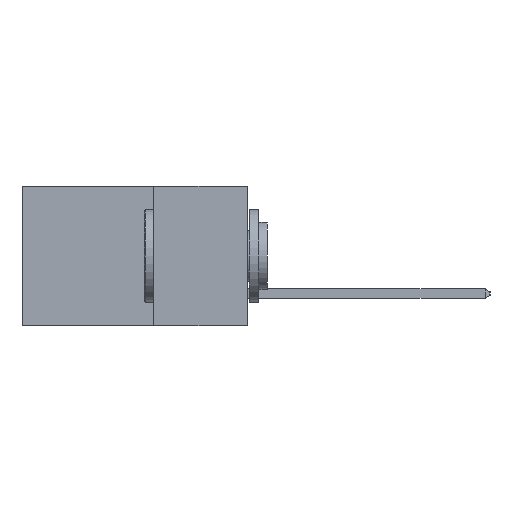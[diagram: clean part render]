
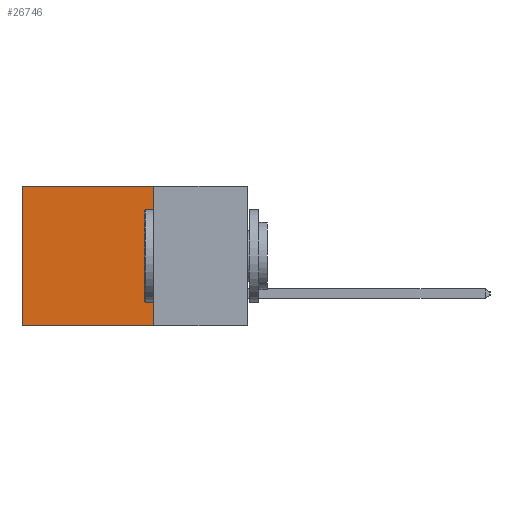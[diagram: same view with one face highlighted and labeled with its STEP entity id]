
A CAD part, left-side view. The second image highlights one B-rep face of the part: STEP entity #26746.
In plain terms, the highlighted planar face has unit normal (-1, 0, 0).
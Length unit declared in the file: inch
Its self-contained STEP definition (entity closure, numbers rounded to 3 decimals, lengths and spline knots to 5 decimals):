
#23 = VECTOR ( 'NONE', #11287, 39.37008 ) ;
#292 = EDGE_CURVE ( 'NONE', #16290, #5317, #12452, .T. ) ;
#1235 = FACE_OUTER_BOUND ( 'NONE', #13264, .T. ) ;
#2104 = CARTESIAN_POINT ( 'NONE',  ( 0.298, 0.6, 0. ) ) ;
#3529 = AXIS2_PLACEMENT_3D ( 'NONE', #7852, #22673, #10129 ) ;
#3675 = ORIENTED_EDGE ( 'NONE', *, *, #27439, .T. ) ;
#3745 = CARTESIAN_POINT ( 'NONE',  ( 0.298, 0.25, 0. ) ) ;
#4123 = VERTEX_POINT ( 'NONE', #21171 ) ;
#5091 = CARTESIAN_POINT ( 'NONE',  ( 0.298, 0.25, 0. ) ) ;
#5317 = VERTEX_POINT ( 'NONE', #16484 ) ;
#7852 = CARTESIAN_POINT ( 'NONE',  ( 0.298, 0.25, 0. ) ) ;
#8491 = CARTESIAN_POINT ( 'NONE',  ( 0.298, 0.25, -0.37 ) ) ;
#8669 = CARTESIAN_POINT ( 'NONE',  ( 0.298, 0.6, 0. ) ) ;
#10129 = DIRECTION ( 'NONE',  ( 0., 0., -1. ) ) ;
#10867 = DIRECTION ( 'NONE',  ( 0., 0., -1. ) ) ;
#11287 = DIRECTION ( 'NONE',  ( 0., 1., 0. ) ) ;
#12452 = LINE ( 'NONE', #8491, #23 ) ;
#12669 = LINE ( 'NONE', #8669, #23038 ) ;
#13264 = EDGE_LOOP ( 'NONE', ( #13481, #19899, #25701, #3675 ) ) ;
#13481 = ORIENTED_EDGE ( 'NONE', *, *, #18320, .T. ) ;
#13655 = CARTESIAN_POINT ( 'NONE',  ( 0.298, 0.25, -0.37 ) ) ;
#14613 = DIRECTION ( 'NONE',  ( 0., 1., 0. ) ) ;
#16290 = VERTEX_POINT ( 'NONE', #13655 ) ;
#16346 = EDGE_CURVE ( 'NONE', #4123, #16290, #21830, .T. ) ;
#16478 = PLANE ( 'NONE',  #3529 ) ;
#16484 = CARTESIAN_POINT ( 'NONE',  ( 0.298, 0.6, -0.37 ) ) ;
#18320 = EDGE_CURVE ( 'NONE', #25678, #5317, #12669, .T. ) ;
#19899 = ORIENTED_EDGE ( 'NONE', *, *, #292, .F. ) ;
#21016 = LINE ( 'NONE', #3745, #25879 ) ;
#21171 = CARTESIAN_POINT ( 'NONE',  ( 0.298, 0.25, 0. ) ) ;
#21830 = LINE ( 'NONE', #5091, #26062 ) ;
#22058 = DIRECTION ( 'NONE',  ( 0., 0., -1. ) ) ;
#22673 = DIRECTION ( 'NONE',  ( 1., 0., 0. ) ) ;
#23038 = VECTOR ( 'NONE', #10867, 39.37008 ) ;
#25678 = VERTEX_POINT ( 'NONE', #2104 ) ;
#25701 = ORIENTED_EDGE ( 'NONE', *, *, #16346, .F. ) ;
#25879 = VECTOR ( 'NONE', #14613, 39.37008 ) ;
#26062 = VECTOR ( 'NONE', #22058, 39.37008 ) ;
#26746 = ADVANCED_FACE ( 'NONE', ( #1235 ), #16478, .F. ) ;
#27439 = EDGE_CURVE ( 'NONE', #4123, #25678, #21016, .T. ) ;
